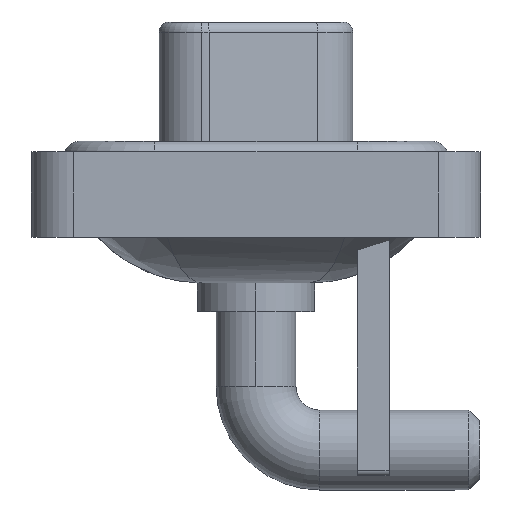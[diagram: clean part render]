
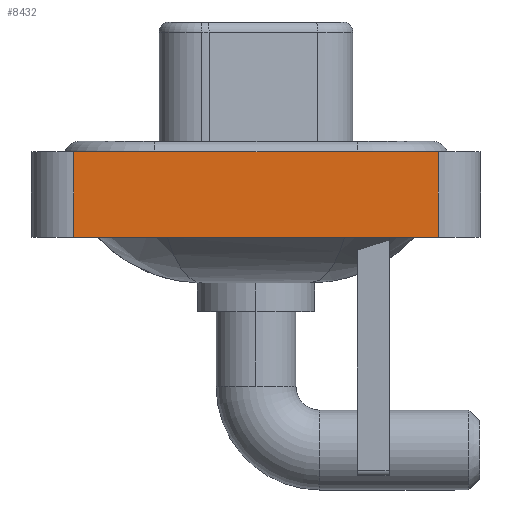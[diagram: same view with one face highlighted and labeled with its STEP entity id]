
A CAD part, left-side view. The second image highlights one B-rep face of the part: STEP entity #8432.
In plain terms, the highlighted planar face has unit normal (-1, 0, 0).
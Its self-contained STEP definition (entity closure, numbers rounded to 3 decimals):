
#273 = ORIENTED_EDGE ( 'NONE', *, *, #2144, .T. ) ;
#1187 = VECTOR ( 'NONE', #12107, 1000. ) ;
#1218 = CARTESIAN_POINT ( 'NONE',  ( -7.25, 8.55, -3.6 ) ) ;
#1360 = EDGE_CURVE ( 'NONE', #5401, #17050, #15457, .T. ) ;
#2144 = EDGE_CURVE ( 'NONE', #17050, #13475, #16177, .T. ) ;
#3271 = CARTESIAN_POINT ( 'NONE',  ( -7.25, -8.55, -3.6 ) ) ;
#3778 = CARTESIAN_POINT ( 'NONE',  ( -7.25, -8.55, -3.6 ) ) ;
#4567 = ORIENTED_EDGE ( 'NONE', *, *, #9629, .F. ) ;
#4668 = CARTESIAN_POINT ( 'NONE',  ( -7.25, 8.55, -3.6 ) ) ;
#5210 = LINE ( 'NONE', #10558, #14995 ) ;
#5401 = VERTEX_POINT ( 'NONE', #1218 ) ;
#5854 = DIRECTION ( 'NONE',  ( -1., 0., 0. ) ) ;
#6435 = DIRECTION ( 'NONE',  ( 0., -1., 0. ) ) ;
#6804 = DIRECTION ( 'NONE',  ( 0., -1., 0. ) ) ;
#8432 = ADVANCED_FACE ( 'NONE', ( #11379 ), #14210, .T. ) ;
#8850 = CARTESIAN_POINT ( 'NONE',  ( -7.25, 8.55, 0.4 ) ) ;
#8930 = EDGE_CURVE ( 'NONE', #5401, #15608, #15965, .T. ) ;
#9244 = AXIS2_PLACEMENT_3D ( 'NONE', #3778, #5854, #17776 ) ;
#9292 = VECTOR ( 'NONE', #6804, 1000. ) ;
#9544 = CARTESIAN_POINT ( 'NONE',  ( -7.25, -8.55, 0.4 ) ) ;
#9629 = EDGE_CURVE ( 'NONE', #15608, #13475, #5210, .T. ) ;
#10202 = CARTESIAN_POINT ( 'NONE',  ( -7.25, -8.55, -3.6 ) ) ;
#10558 = CARTESIAN_POINT ( 'NONE',  ( -7.25, -8.55, 0.4 ) ) ;
#11017 = CARTESIAN_POINT ( 'NONE',  ( -7.25, -8.55, -3.6 ) ) ;
#11379 = FACE_OUTER_BOUND ( 'NONE', #12843, .T. ) ;
#12107 = DIRECTION ( 'NONE',  ( 0., 0., 1. ) ) ;
#12843 = EDGE_LOOP ( 'NONE', ( #273, #4567, #18586, #16713 ) ) ;
#13035 = DIRECTION ( 'NONE',  ( 0., 0., 1. ) ) ;
#13475 = VERTEX_POINT ( 'NONE', #9544 ) ;
#14210 = PLANE ( 'NONE',  #9244 ) ;
#14995 = VECTOR ( 'NONE', #6435, 1000. ) ;
#15457 = LINE ( 'NONE', #11017, #9292 ) ;
#15608 = VERTEX_POINT ( 'NONE', #8850 ) ;
#15965 = LINE ( 'NONE', #4668, #17711 ) ;
#16177 = LINE ( 'NONE', #3271, #1187 ) ;
#16713 = ORIENTED_EDGE ( 'NONE', *, *, #1360, .T. ) ;
#17050 = VERTEX_POINT ( 'NONE', #10202 ) ;
#17711 = VECTOR ( 'NONE', #13035, 1000. ) ;
#17776 = DIRECTION ( 'NONE',  ( 0., 0., 1. ) ) ;
#18586 = ORIENTED_EDGE ( 'NONE', *, *, #8930, .F. ) ;
